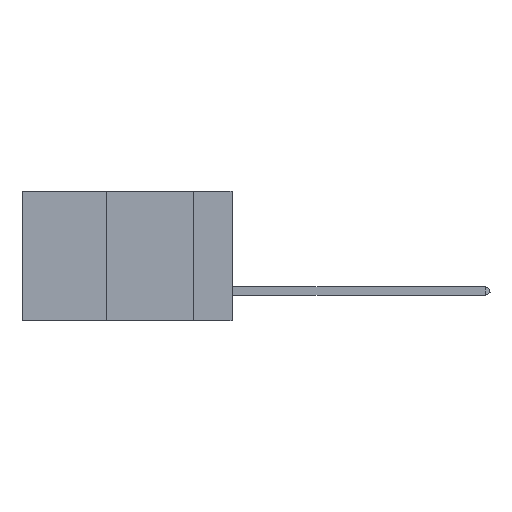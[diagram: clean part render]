
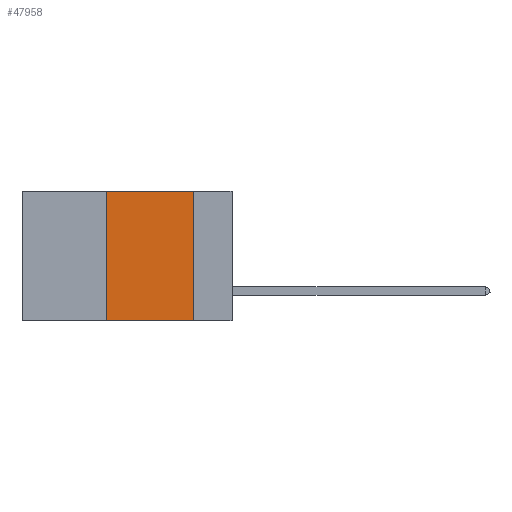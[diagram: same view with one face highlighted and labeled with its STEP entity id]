
A CAD part, left-side view. The second image highlights one B-rep face of the part: STEP entity #47958.
In plain terms, the highlighted planar face has unit normal (-1, 0, 0).
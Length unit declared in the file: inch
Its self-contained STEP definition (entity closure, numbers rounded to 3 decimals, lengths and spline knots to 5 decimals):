
#836 = LINE ( 'NONE', #40949, #34763 ) ;
#5256 = AXIS2_PLACEMENT_3D ( 'NONE', #5708, #20427, #24150 ) ;
#5708 = CARTESIAN_POINT ( 'NONE',  ( 0., 0.6, 0. ) ) ;
#6183 = ORIENTED_EDGE ( 'NONE', *, *, #30615, .T. ) ;
#6333 = CARTESIAN_POINT ( 'NONE',  ( 0., 0.6, -0.37 ) ) ;
#7136 = VECTOR ( 'NONE', #12541, 39.37008 ) ;
#8281 = LINE ( 'NONE', #37496, #30541 ) ;
#8418 = CARTESIAN_POINT ( 'NONE',  ( 0., 0.36, 0. ) ) ;
#9705 = ORIENTED_EDGE ( 'NONE', *, *, #46455, .F. ) ;
#9885 = CARTESIAN_POINT ( 'NONE',  ( 0., 0.36, 0. ) ) ;
#12384 = ORIENTED_EDGE ( 'NONE', *, *, #22638, .F. ) ;
#12541 = DIRECTION ( 'NONE',  ( 0., 0., 1. ) ) ;
#15450 = ORIENTED_EDGE ( 'NONE', *, *, #18130, .F. ) ;
#16497 = PLANE ( 'NONE',  #5256 ) ;
#18130 = EDGE_CURVE ( 'NONE', #20888, #28923, #8281, .T. ) ;
#19620 = VERTEX_POINT ( 'NONE', #25529 ) ;
#20427 = DIRECTION ( 'NONE',  ( 1., 0., 0. ) ) ;
#20888 = VERTEX_POINT ( 'NONE', #47461 ) ;
#21601 = CARTESIAN_POINT ( 'NONE',  ( 0., 0.11, -0.37 ) ) ;
#21706 = DIRECTION ( 'NONE',  ( 0., -1., 0. ) ) ;
#22638 = EDGE_CURVE ( 'NONE', #19620, #45558, #37584, .T. ) ;
#24150 = DIRECTION ( 'NONE',  ( 0., 0., -1. ) ) ;
#25529 = CARTESIAN_POINT ( 'NONE',  ( 0., 0.36, -0.37 ) ) ;
#27228 = LINE ( 'NONE', #6333, #38450 ) ;
#28923 = VERTEX_POINT ( 'NONE', #21601 ) ;
#30541 = VECTOR ( 'NONE', #41393, 39.37008 ) ;
#30615 = EDGE_CURVE ( 'NONE', #19620, #28923, #27228, .T. ) ;
#34763 = VECTOR ( 'NONE', #36867, 39.37008 ) ;
#35207 = FACE_OUTER_BOUND ( 'NONE', #40223, .T. ) ;
#36867 = DIRECTION ( 'NONE',  ( 0., -1., 0. ) ) ;
#37496 = CARTESIAN_POINT ( 'NONE',  ( 0., 0.11, 0. ) ) ;
#37584 = LINE ( 'NONE', #8418, #7136 ) ;
#38450 = VECTOR ( 'NONE', #21706, 39.37008 ) ;
#40223 = EDGE_LOOP ( 'NONE', ( #15450, #9705, #12384, #6183 ) ) ;
#40949 = CARTESIAN_POINT ( 'NONE',  ( 0., 0.6, 0. ) ) ;
#41393 = DIRECTION ( 'NONE',  ( 0., 0., -1. ) ) ;
#45558 = VERTEX_POINT ( 'NONE', #9885 ) ;
#46455 = EDGE_CURVE ( 'NONE', #45558, #20888, #836, .T. ) ;
#47461 = CARTESIAN_POINT ( 'NONE',  ( 0., 0.11, 0. ) ) ;
#47958 = ADVANCED_FACE ( 'NONE', ( #35207 ), #16497, .F. ) ;
